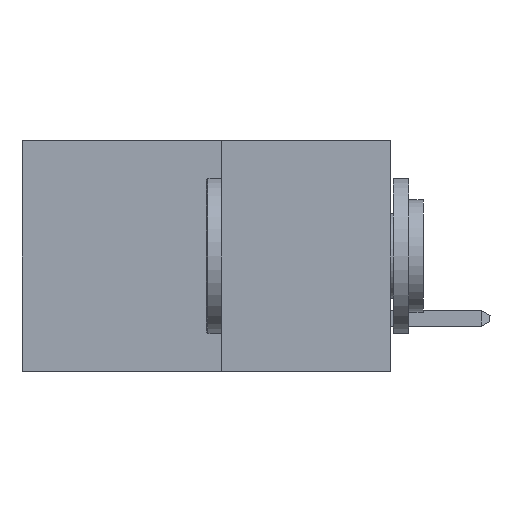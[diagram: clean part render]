
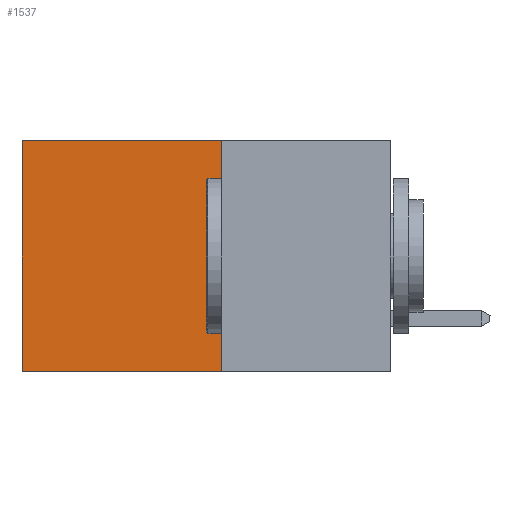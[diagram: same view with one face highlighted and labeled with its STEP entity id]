
A CAD part, left-side view. The second image highlights one B-rep face of the part: STEP entity #1537.
In plain terms, the highlighted planar face has unit normal (-1, 0, 0).
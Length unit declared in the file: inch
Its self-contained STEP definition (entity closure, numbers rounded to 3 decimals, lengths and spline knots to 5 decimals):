
#283 = VERTEX_POINT ( 'NONE', #17600 ) ;
#1107 = EDGE_CURVE ( 'NONE', #3775, #14700, #9642, .T. ) ;
#1537 = ADVANCED_FACE ( 'NONE', ( #15473 ), #15798, .F. ) ;
#2049 = CARTESIAN_POINT ( 'NONE',  ( 0.277, 0.27, -0.37 ) ) ;
#2646 = AXIS2_PLACEMENT_3D ( 'NONE', #6393, #6937, #9413 ) ;
#2950 = DIRECTION ( 'NONE',  ( 0., 1., 0. ) ) ;
#3775 = VERTEX_POINT ( 'NONE', #5974 ) ;
#4538 = EDGE_CURVE ( 'NONE', #19250, #283, #20408, .T. ) ;
#4646 = CARTESIAN_POINT ( 'NONE',  ( 0.277, 0.27, 0. ) ) ;
#5974 = CARTESIAN_POINT ( 'NONE',  ( 0.277, 0.59, 0. ) ) ;
#6131 = ORIENTED_EDGE ( 'NONE', *, *, #4538, .F. ) ;
#6393 = CARTESIAN_POINT ( 'NONE',  ( 0.277, 0.27, -0.37 ) ) ;
#6493 = ORIENTED_EDGE ( 'NONE', *, *, #1107, .T. ) ;
#6937 = DIRECTION ( 'NONE',  ( 1., 0., 0. ) ) ;
#7496 = VECTOR ( 'NONE', #8699, 39.37008 ) ;
#7841 = EDGE_LOOP ( 'NONE', ( #6493, #15238, #6131, #17121 ) ) ;
#8699 = DIRECTION ( 'NONE',  ( 0., 1., 0. ) ) ;
#9363 = EDGE_CURVE ( 'NONE', #283, #14700, #15354, .T. ) ;
#9413 = DIRECTION ( 'NONE',  ( 0., 0., -1. ) ) ;
#9571 = CARTESIAN_POINT ( 'NONE',  ( 0.277, 0.59, -0.37 ) ) ;
#9642 = LINE ( 'NONE', #9990, #17463 ) ;
#9990 = CARTESIAN_POINT ( 'NONE',  ( 0.277, 0.59, -0.37 ) ) ;
#11273 = LINE ( 'NONE', #13994, #14898 ) ;
#11424 = DIRECTION ( 'NONE',  ( 0., 0., -1. ) ) ;
#12242 = VECTOR ( 'NONE', #14673, 39.37008 ) ;
#13474 = CARTESIAN_POINT ( 'NONE',  ( 0.277, 0.27, -0.37 ) ) ;
#13994 = CARTESIAN_POINT ( 'NONE',  ( 0.277, 0.27, 0. ) ) ;
#14673 = DIRECTION ( 'NONE',  ( 0., 0., -1. ) ) ;
#14700 = VERTEX_POINT ( 'NONE', #9571 ) ;
#14898 = VECTOR ( 'NONE', #2950, 39.37008 ) ;
#15238 = ORIENTED_EDGE ( 'NONE', *, *, #9363, .F. ) ;
#15354 = LINE ( 'NONE', #13474, #7496 ) ;
#15473 = FACE_OUTER_BOUND ( 'NONE', #7841, .T. ) ;
#15798 = PLANE ( 'NONE',  #2646 ) ;
#17121 = ORIENTED_EDGE ( 'NONE', *, *, #17895, .T. ) ;
#17463 = VECTOR ( 'NONE', #11424, 39.37008 ) ;
#17600 = CARTESIAN_POINT ( 'NONE',  ( 0.277, 0.27, -0.37 ) ) ;
#17895 = EDGE_CURVE ( 'NONE', #19250, #3775, #11273, .T. ) ;
#19250 = VERTEX_POINT ( 'NONE', #4646 ) ;
#20408 = LINE ( 'NONE', #2049, #12242 ) ;
